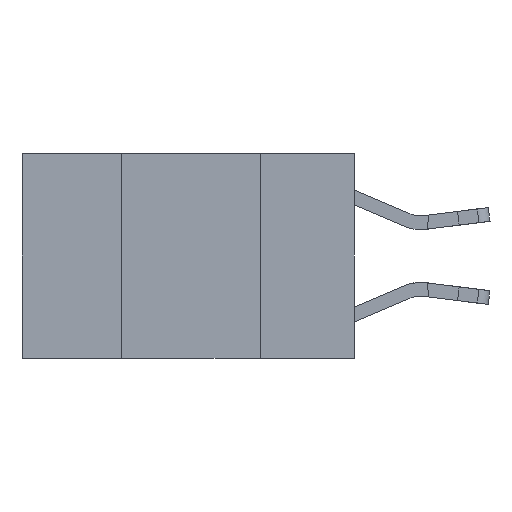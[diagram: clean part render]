
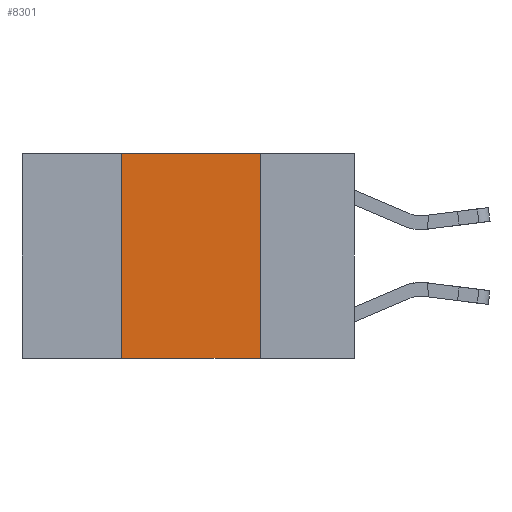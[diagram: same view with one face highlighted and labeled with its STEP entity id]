
A CAD part, left-side view. The second image highlights one B-rep face of the part: STEP entity #8301.
In plain terms, the highlighted planar face has unit normal (-1, 0, 0).
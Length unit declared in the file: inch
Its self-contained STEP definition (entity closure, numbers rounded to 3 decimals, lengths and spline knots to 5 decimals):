
#394 = CARTESIAN_POINT ( 'NONE',  ( 0., 0.17, 0. ) ) ;
#1444 = ORIENTED_EDGE ( 'NONE', *, *, #20359, .T. ) ;
#1477 = CARTESIAN_POINT ( 'NONE',  ( 0., 0.17, 0. ) ) ;
#1878 = ORIENTED_EDGE ( 'NONE', *, *, #21621, .F. ) ;
#2569 = CARTESIAN_POINT ( 'NONE',  ( 0., 0.6, 0. ) ) ;
#3619 = CARTESIAN_POINT ( 'NONE',  ( 0., 0.42, -0.37 ) ) ;
#3956 = VERTEX_POINT ( 'NONE', #13858 ) ;
#4538 = DIRECTION ( 'NONE',  ( 1., 0., 0. ) ) ;
#5281 = VERTEX_POINT ( 'NONE', #3619 ) ;
#7199 = PLANE ( 'NONE',  #16267 ) ;
#8301 = ADVANCED_FACE ( 'NONE', ( #8876 ), #7199, .F. ) ;
#8876 = FACE_OUTER_BOUND ( 'NONE', #14701, .T. ) ;
#10168 = VECTOR ( 'NONE', #15135, 39.37008 ) ;
#11492 = ORIENTED_EDGE ( 'NONE', *, *, #26847, .F. ) ;
#11959 = VECTOR ( 'NONE', #21759, 39.37008 ) ;
#12641 = VERTEX_POINT ( 'NONE', #23749 ) ;
#13312 = LINE ( 'NONE', #17252, #11959 ) ;
#13858 = CARTESIAN_POINT ( 'NONE',  ( 0., 0.17, -0.37 ) ) ;
#14701 = EDGE_LOOP ( 'NONE', ( #23092, #1878, #11492, #1444 ) ) ;
#15135 = DIRECTION ( 'NONE',  ( 0., 0., 1. ) ) ;
#15451 = LINE ( 'NONE', #394, #26797 ) ;
#16267 = AXIS2_PLACEMENT_3D ( 'NONE', #2569, #4538, #17747 ) ;
#16616 = LINE ( 'NONE', #22815, #19181 ) ;
#17252 = CARTESIAN_POINT ( 'NONE',  ( 0., 0.6, -0.37 ) ) ;
#17621 = VERTEX_POINT ( 'NONE', #1477 ) ;
#17747 = DIRECTION ( 'NONE',  ( 0., 0., -1. ) ) ;
#18447 = DIRECTION ( 'NONE',  ( 0., -1., 0. ) ) ;
#19181 = VECTOR ( 'NONE', #18447, 39.37008 ) ;
#19880 = EDGE_CURVE ( 'NONE', #17621, #3956, #15451, .T. ) ;
#20359 = EDGE_CURVE ( 'NONE', #5281, #3956, #13312, .T. ) ;
#21615 = CARTESIAN_POINT ( 'NONE',  ( 0., 0.42, 0. ) ) ;
#21621 = EDGE_CURVE ( 'NONE', #12641, #17621, #16616, .T. ) ;
#21759 = DIRECTION ( 'NONE',  ( 0., -1., 0. ) ) ;
#22161 = LINE ( 'NONE', #21615, #10168 ) ;
#22815 = CARTESIAN_POINT ( 'NONE',  ( 0., 0.6, 0. ) ) ;
#23092 = ORIENTED_EDGE ( 'NONE', *, *, #19880, .F. ) ;
#23749 = CARTESIAN_POINT ( 'NONE',  ( 0., 0.42, 0. ) ) ;
#25746 = DIRECTION ( 'NONE',  ( 0., 0., -1. ) ) ;
#26797 = VECTOR ( 'NONE', #25746, 39.37008 ) ;
#26847 = EDGE_CURVE ( 'NONE', #5281, #12641, #22161, .T. ) ;
